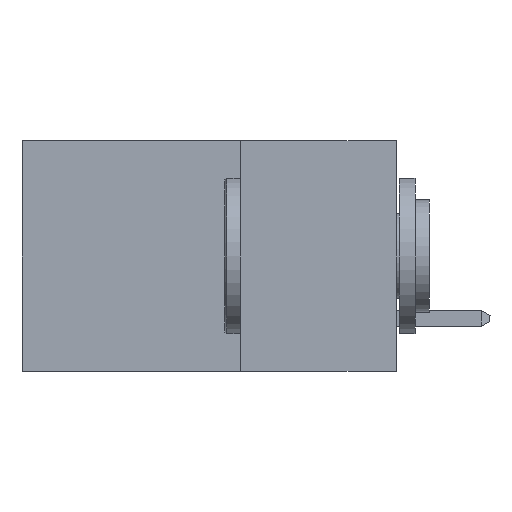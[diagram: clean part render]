
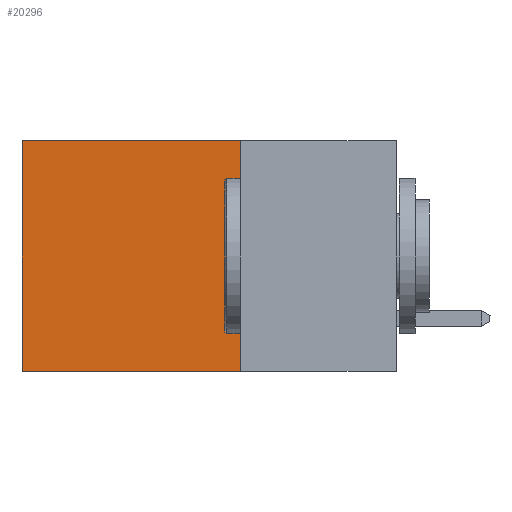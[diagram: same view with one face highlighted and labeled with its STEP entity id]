
A CAD part, left-side view. The second image highlights one B-rep face of the part: STEP entity #20296.
In plain terms, the highlighted planar face has unit normal (-1, 0, 0).
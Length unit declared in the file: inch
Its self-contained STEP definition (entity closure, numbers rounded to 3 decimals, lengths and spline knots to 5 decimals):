
#652 = VECTOR ( 'NONE', #10245, 39.37008 ) ;
#1824 = CARTESIAN_POINT ( 'NONE',  ( 0.2615, 0.6, -0.37 ) ) ;
#1851 = DIRECTION ( 'NONE',  ( 0., 0., -1. ) ) ;
#2183 = VECTOR ( 'NONE', #15184, 39.37008 ) ;
#2311 = VECTOR ( 'NONE', #1851, 39.37008 ) ;
#2816 = LINE ( 'NONE', #1824, #2311 ) ;
#3376 = VERTEX_POINT ( 'NONE', #9512 ) ;
#5026 = DIRECTION ( 'NONE',  ( 0., 0., -1. ) ) ;
#5335 = LINE ( 'NONE', #8829, #18089 ) ;
#5585 = CARTESIAN_POINT ( 'NONE',  ( 0.2615, 0.25, -0.37 ) ) ;
#6129 = VERTEX_POINT ( 'NONE', #10041 ) ;
#6312 = LINE ( 'NONE', #5585, #2183 ) ;
#6905 = VERTEX_POINT ( 'NONE', #10160 ) ;
#8104 = EDGE_CURVE ( 'NONE', #8654, #6129, #2816, .T. ) ;
#8654 = VERTEX_POINT ( 'NONE', #16416 ) ;
#8829 = CARTESIAN_POINT ( 'NONE',  ( 0.2615, 0.25, 0. ) ) ;
#9512 = CARTESIAN_POINT ( 'NONE',  ( 0.2615, 0.25, 0. ) ) ;
#10041 = CARTESIAN_POINT ( 'NONE',  ( 0.2615, 0.6, -0.37 ) ) ;
#10160 = CARTESIAN_POINT ( 'NONE',  ( 0.2615, 0.25, -0.37 ) ) ;
#10172 = CARTESIAN_POINT ( 'NONE',  ( 0.2615, 0.25, -0.37 ) ) ;
#10245 = DIRECTION ( 'NONE',  ( 0., 1., 0. ) ) ;
#10301 = EDGE_LOOP ( 'NONE', ( #18318, #15296, #14819, #12903 ) ) ;
#11327 = PLANE ( 'NONE',  #13255 ) ;
#12903 = ORIENTED_EDGE ( 'NONE', *, *, #16571, .T. ) ;
#12978 = CARTESIAN_POINT ( 'NONE',  ( 0.2615, 0.25, -0.37 ) ) ;
#13255 = AXIS2_PLACEMENT_3D ( 'NONE', #12978, #14593, #5026 ) ;
#13411 = LINE ( 'NONE', #10172, #652 ) ;
#14593 = DIRECTION ( 'NONE',  ( 1., 0., 0. ) ) ;
#14819 = ORIENTED_EDGE ( 'NONE', *, *, #16544, .F. ) ;
#15184 = DIRECTION ( 'NONE',  ( 0., 0., -1. ) ) ;
#15296 = ORIENTED_EDGE ( 'NONE', *, *, #20514, .F. ) ;
#16416 = CARTESIAN_POINT ( 'NONE',  ( 0.2615, 0.6, 0. ) ) ;
#16544 = EDGE_CURVE ( 'NONE', #3376, #6905, #6312, .T. ) ;
#16571 = EDGE_CURVE ( 'NONE', #3376, #8654, #5335, .T. ) ;
#17930 = FACE_OUTER_BOUND ( 'NONE', #10301, .T. ) ;
#18089 = VECTOR ( 'NONE', #19934, 39.37008 ) ;
#18318 = ORIENTED_EDGE ( 'NONE', *, *, #8104, .T. ) ;
#19934 = DIRECTION ( 'NONE',  ( 0., 1., 0. ) ) ;
#20296 = ADVANCED_FACE ( 'NONE', ( #17930 ), #11327, .F. ) ;
#20514 = EDGE_CURVE ( 'NONE', #6905, #6129, #13411, .T. ) ;
